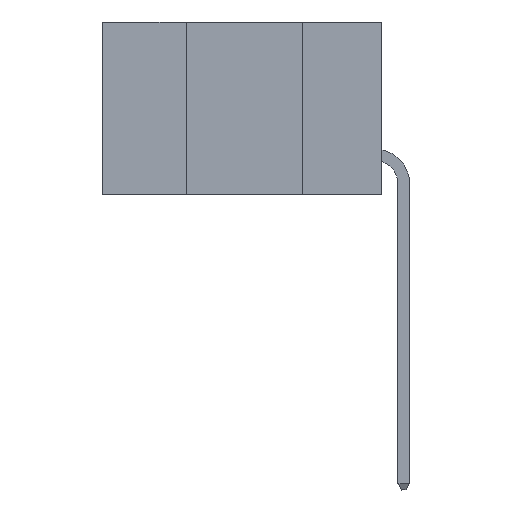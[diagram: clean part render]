
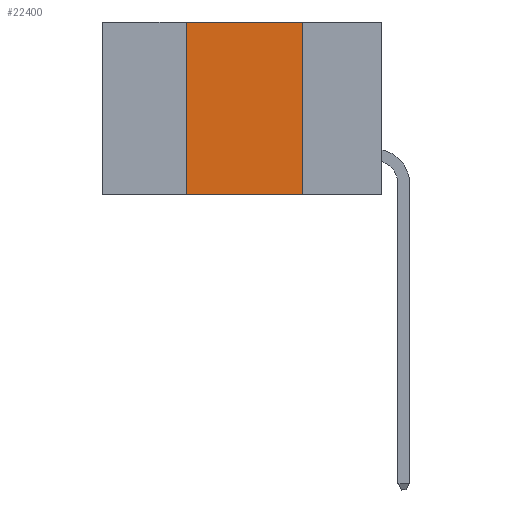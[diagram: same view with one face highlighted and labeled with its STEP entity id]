
A CAD part, left-side view. The second image highlights one B-rep face of the part: STEP entity #22400.
In plain terms, the highlighted planar face has unit normal (-1, 0, 0).
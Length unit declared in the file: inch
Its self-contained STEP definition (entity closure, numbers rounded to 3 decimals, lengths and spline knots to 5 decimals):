
#96 = LINE ( 'NONE', #13919, #2330 ) ;
#624 = CARTESIAN_POINT ( 'NONE',  ( 0., 0.42, -0.37 ) ) ;
#1089 = VECTOR ( 'NONE', #6697, 39.37008 ) ;
#1187 = ORIENTED_EDGE ( 'NONE', *, *, #11935, .T. ) ;
#1530 = DIRECTION ( 'NONE',  ( 0., 0., -1. ) ) ;
#2012 = PLANE ( 'NONE',  #24069 ) ;
#2330 = VECTOR ( 'NONE', #30414, 39.37008 ) ;
#3006 = LINE ( 'NONE', #25433, #1089 ) ;
#6697 = DIRECTION ( 'NONE',  ( 0., -1., 0. ) ) ;
#7315 = VERTEX_POINT ( 'NONE', #28049 ) ;
#7326 = EDGE_CURVE ( 'NONE', #7367, #7315, #96, .T. ) ;
#7367 = VERTEX_POINT ( 'NONE', #9108 ) ;
#8028 = VERTEX_POINT ( 'NONE', #28397 ) ;
#8921 = CARTESIAN_POINT ( 'NONE',  ( 0., 0.6, 0. ) ) ;
#9108 = CARTESIAN_POINT ( 'NONE',  ( 0., 0.42, 0. ) ) ;
#10064 = EDGE_CURVE ( 'NONE', #28838, #7367, #10978, .T. ) ;
#10978 = LINE ( 'NONE', #16521, #11713 ) ;
#11713 = VECTOR ( 'NONE', #13463, 39.37008 ) ;
#11935 = EDGE_CURVE ( 'NONE', #28838, #8028, #3006, .T. ) ;
#13463 = DIRECTION ( 'NONE',  ( 0., 0., 1. ) ) ;
#13475 = LINE ( 'NONE', #20517, #16454 ) ;
#13919 = CARTESIAN_POINT ( 'NONE',  ( 0., 0.6, 0. ) ) ;
#16284 = ORIENTED_EDGE ( 'NONE', *, *, #26556, .F. ) ;
#16454 = VECTOR ( 'NONE', #1530, 39.37008 ) ;
#16521 = CARTESIAN_POINT ( 'NONE',  ( 0., 0.42, 0. ) ) ;
#18410 = DIRECTION ( 'NONE',  ( 0., 0., -1. ) ) ;
#20517 = CARTESIAN_POINT ( 'NONE',  ( 0., 0.17, 0. ) ) ;
#22130 = EDGE_LOOP ( 'NONE', ( #16284, #29576, #25533, #1187 ) ) ;
#22400 = ADVANCED_FACE ( 'NONE', ( #24994 ), #2012, .F. ) ;
#24069 = AXIS2_PLACEMENT_3D ( 'NONE', #8921, #27857, #18410 ) ;
#24994 = FACE_OUTER_BOUND ( 'NONE', #22130, .T. ) ;
#25433 = CARTESIAN_POINT ( 'NONE',  ( 0., 0.6, -0.37 ) ) ;
#25533 = ORIENTED_EDGE ( 'NONE', *, *, #10064, .F. ) ;
#26556 = EDGE_CURVE ( 'NONE', #7315, #8028, #13475, .T. ) ;
#27857 = DIRECTION ( 'NONE',  ( 1., 0., 0. ) ) ;
#28049 = CARTESIAN_POINT ( 'NONE',  ( 0., 0.17, 0. ) ) ;
#28397 = CARTESIAN_POINT ( 'NONE',  ( 0., 0.17, -0.37 ) ) ;
#28838 = VERTEX_POINT ( 'NONE', #624 ) ;
#29576 = ORIENTED_EDGE ( 'NONE', *, *, #7326, .F. ) ;
#30414 = DIRECTION ( 'NONE',  ( 0., -1., 0. ) ) ;
